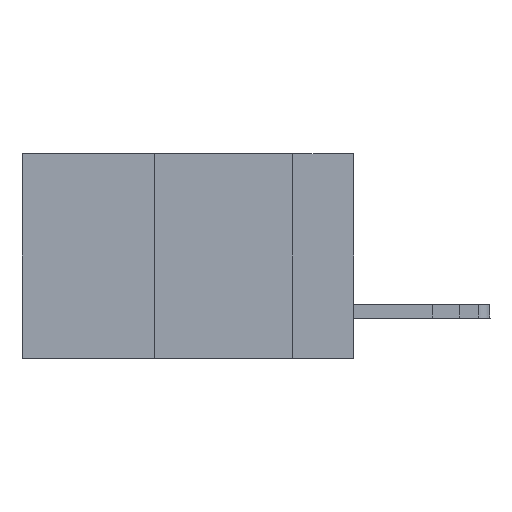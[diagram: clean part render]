
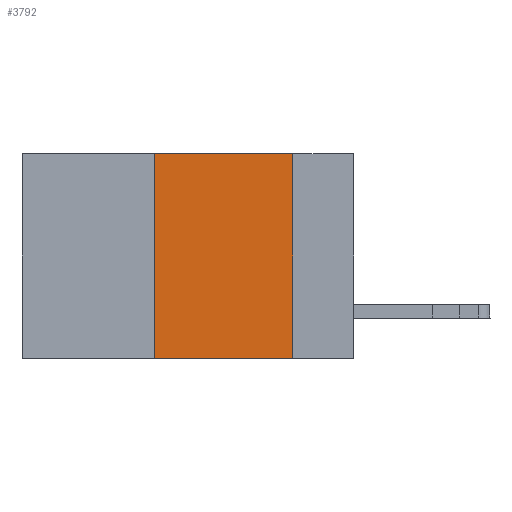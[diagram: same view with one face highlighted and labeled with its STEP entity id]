
A CAD part, left-side view. The second image highlights one B-rep face of the part: STEP entity #3792.
In plain terms, the highlighted planar face has unit normal (-1, 0, 0).
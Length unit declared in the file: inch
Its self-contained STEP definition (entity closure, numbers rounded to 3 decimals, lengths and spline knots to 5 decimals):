
#560 = EDGE_LOOP ( 'NONE', ( #21584, #26211, #33704, #25111 ) ) ;
#943 = PLANE ( 'NONE',  #34665 ) ;
#2545 = DIRECTION ( 'NONE',  ( 0., 0., -1. ) ) ;
#3597 = LINE ( 'NONE', #25566, #5681 ) ;
#3629 = VERTEX_POINT ( 'NONE', #7546 ) ;
#3651 = EDGE_CURVE ( 'NONE', #3629, #26714, #12912, .T. ) ;
#3792 = ADVANCED_FACE ( 'NONE', ( #27947 ), #943, .F. ) ;
#4444 = LINE ( 'NONE', #28417, #17053 ) ;
#5442 = VERTEX_POINT ( 'NONE', #21475 ) ;
#5681 = VECTOR ( 'NONE', #31632, 39.37008 ) ;
#7415 = EDGE_CURVE ( 'NONE', #22945, #26714, #4444, .T. ) ;
#7546 = CARTESIAN_POINT ( 'NONE',  ( 0., 0.11, 0. ) ) ;
#10532 = CARTESIAN_POINT ( 'NONE',  ( 0., 0.36, -0.37 ) ) ;
#10661 = VECTOR ( 'NONE', #27419, 39.37008 ) ;
#11501 = CARTESIAN_POINT ( 'NONE',  ( 0., 0.6, 0. ) ) ;
#11675 = DIRECTION ( 'NONE',  ( 0., 0., -1. ) ) ;
#12912 = LINE ( 'NONE', #15968, #28384 ) ;
#15968 = CARTESIAN_POINT ( 'NONE',  ( 0., 0.11, 0. ) ) ;
#17053 = VECTOR ( 'NONE', #21055, 39.37008 ) ;
#18890 = CARTESIAN_POINT ( 'NONE',  ( 0., 0.11, -0.37 ) ) ;
#21055 = DIRECTION ( 'NONE',  ( 0., -1., 0. ) ) ;
#21475 = CARTESIAN_POINT ( 'NONE',  ( 0., 0.36, 0. ) ) ;
#21584 = ORIENTED_EDGE ( 'NONE', *, *, #3651, .F. ) ;
#22945 = VERTEX_POINT ( 'NONE', #10532 ) ;
#25111 = ORIENTED_EDGE ( 'NONE', *, *, #7415, .T. ) ;
#25566 = CARTESIAN_POINT ( 'NONE',  ( 0., 0.6, 0. ) ) ;
#25784 = EDGE_CURVE ( 'NONE', #22945, #5442, #34947, .T. ) ;
#26211 = ORIENTED_EDGE ( 'NONE', *, *, #34272, .F. ) ;
#26714 = VERTEX_POINT ( 'NONE', #18890 ) ;
#27419 = DIRECTION ( 'NONE',  ( 0., 0., 1. ) ) ;
#27947 = FACE_OUTER_BOUND ( 'NONE', #560, .T. ) ;
#28384 = VECTOR ( 'NONE', #2545, 39.37008 ) ;
#28417 = CARTESIAN_POINT ( 'NONE',  ( 0., 0.6, -0.37 ) ) ;
#29745 = CARTESIAN_POINT ( 'NONE',  ( 0., 0.36, 0. ) ) ;
#30270 = DIRECTION ( 'NONE',  ( 1., 0., 0. ) ) ;
#31632 = DIRECTION ( 'NONE',  ( 0., -1., 0. ) ) ;
#33704 = ORIENTED_EDGE ( 'NONE', *, *, #25784, .F. ) ;
#34272 = EDGE_CURVE ( 'NONE', #5442, #3629, #3597, .T. ) ;
#34665 = AXIS2_PLACEMENT_3D ( 'NONE', #11501, #30270, #11675 ) ;
#34947 = LINE ( 'NONE', #29745, #10661 ) ;
